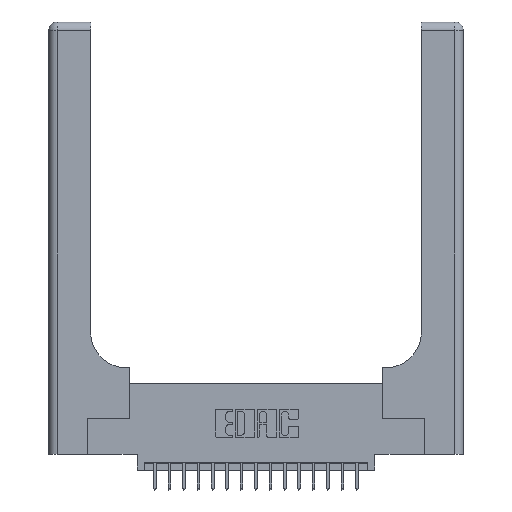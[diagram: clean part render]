
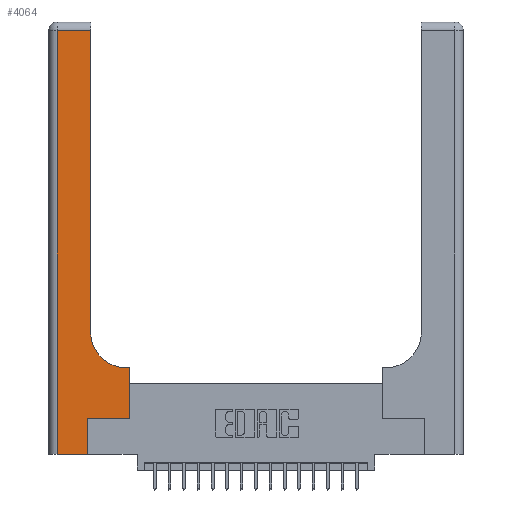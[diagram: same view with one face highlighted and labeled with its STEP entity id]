
A CAD part, top view. The second image highlights one B-rep face of the part: STEP entity #4064.
In plain terms, the highlighted planar face has unit normal (0, 0, 1).
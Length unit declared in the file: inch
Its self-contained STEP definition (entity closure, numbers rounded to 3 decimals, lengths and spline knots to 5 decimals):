
#77 = DIRECTION ( 'NONE',  ( -1., 0., 0. ) ) ;
#83 = VERTEX_POINT ( 'NONE', #14371 ) ;
#908 = LINE ( 'NONE', #13831, #20661 ) ;
#941 = VERTEX_POINT ( 'NONE', #7114 ) ;
#1025 = DIRECTION ( 'NONE',  ( 1., 0., 0. ) ) ;
#1724 = VECTOR ( 'NONE', #4347, 39.37008 ) ;
#1729 = ORIENTED_EDGE ( 'NONE', *, *, #18147, .T. ) ;
#2887 = VERTEX_POINT ( 'NONE', #5457 ) ;
#3178 = CIRCLE ( 'NONE', #10839, 0.25 ) ;
#3492 = CARTESIAN_POINT ( 'NONE',  ( 0.06, 0., 0.37 ) ) ;
#3884 = EDGE_CURVE ( 'NONE', #2887, #7071, #908, .T. ) ;
#3934 = DIRECTION ( 'NONE',  ( -1., 0., 0. ) ) ;
#4064 = ADVANCED_FACE ( 'NONE', ( #6858 ), #6968, .F. ) ;
#4347 = DIRECTION ( 'NONE',  ( 0., -1., 0. ) ) ;
#4430 = LINE ( 'NONE', #17370, #19109 ) ;
#4970 = DIRECTION ( 'NONE',  ( 1., 0., 0. ) ) ;
#5030 = CARTESIAN_POINT ( 'NONE',  ( 0.269, 0., 0.37 ) ) ;
#5044 = VECTOR ( 'NONE', #7420, 39.37008 ) ;
#5072 = CARTESIAN_POINT ( 'NONE',  ( 0.5585, 0.25, 0.37 ) ) ;
#5457 = CARTESIAN_POINT ( 'NONE',  ( 0.2915, 0.85, 0.37 ) ) ;
#5660 = EDGE_CURVE ( 'NONE', #83, #2887, #3178, .T. ) ;
#6353 = DIRECTION ( 'NONE',  ( 1., 0., 0. ) ) ;
#6858 = FACE_OUTER_BOUND ( 'NONE', #18296, .T. ) ;
#6968 = PLANE ( 'NONE',  #12203 ) ;
#7071 = VERTEX_POINT ( 'NONE', #13636 ) ;
#7099 = CARTESIAN_POINT ( 'NONE',  ( 0.5585, 0.6, 0.37 ) ) ;
#7114 = CARTESIAN_POINT ( 'NONE',  ( 0.269, 0., 0.37 ) ) ;
#7201 = CARTESIAN_POINT ( 'NONE',  ( 0.269, 0.25, 0.37 ) ) ;
#7228 = CARTESIAN_POINT ( 'NONE',  ( 0.5585, 0.25, 0.37 ) ) ;
#7420 = DIRECTION ( 'NONE',  ( 0., 1., 0. ) ) ;
#7601 = VECTOR ( 'NONE', #4970, 39.37008 ) ;
#8092 = CARTESIAN_POINT ( 'NONE',  ( 0.269, 0.25, 0.37 ) ) ;
#8152 = VECTOR ( 'NONE', #6353, 39.37008 ) ;
#8417 = ORIENTED_EDGE ( 'NONE', *, *, #9094, .T. ) ;
#9094 = EDGE_CURVE ( 'NONE', #11889, #12499, #9979, .T. ) ;
#9818 = DIRECTION ( 'NONE',  ( 0., 1., 0. ) ) ;
#9979 = LINE ( 'NONE', #8092, #7601 ) ;
#10362 = LINE ( 'NONE', #7228, #5044 ) ;
#10834 = CARTESIAN_POINT ( 'NONE',  ( 0.06, 2.94, 0.37 ) ) ;
#10839 = AXIS2_PLACEMENT_3D ( 'NONE', #18792, #12254, #1025 ) ;
#10935 = EDGE_CURVE ( 'NONE', #941, #11889, #13431, .T. ) ;
#11307 = ORIENTED_EDGE ( 'NONE', *, *, #3884, .T. ) ;
#11318 = VECTOR ( 'NONE', #9818, 39.37008 ) ;
#11889 = VERTEX_POINT ( 'NONE', #7201 ) ;
#11998 = ORIENTED_EDGE ( 'NONE', *, *, #13806, .T. ) ;
#12048 = ORIENTED_EDGE ( 'NONE', *, *, #18334, .T. ) ;
#12203 = AXIS2_PLACEMENT_3D ( 'NONE', #16662, #19724, #3934 ) ;
#12254 = DIRECTION ( 'NONE',  ( 0., 0., -1. ) ) ;
#12499 = VERTEX_POINT ( 'NONE', #5072 ) ;
#12564 = EDGE_CURVE ( 'NONE', #12499, #13043, #10362, .T. ) ;
#13043 = VERTEX_POINT ( 'NONE', #7099 ) ;
#13101 = CARTESIAN_POINT ( 'NONE',  ( 0., 2.94, 0.37 ) ) ;
#13136 = EDGE_CURVE ( 'NONE', #16213, #941, #18883, .T. ) ;
#13431 = LINE ( 'NONE', #5030, #11318 ) ;
#13636 = CARTESIAN_POINT ( 'NONE',  ( 0.2915, 2.94, 0.37 ) ) ;
#13804 = LINE ( 'NONE', #18660, #1724 ) ;
#13806 = EDGE_CURVE ( 'NONE', #13043, #83, #4430, .T. ) ;
#13831 = CARTESIAN_POINT ( 'NONE',  ( 0.2915, 3., 0.37 ) ) ;
#14371 = CARTESIAN_POINT ( 'NONE',  ( 0.5415, 0.6, 0.37 ) ) ;
#14786 = LINE ( 'NONE', #13101, #18176 ) ;
#15641 = ORIENTED_EDGE ( 'NONE', *, *, #12564, .T. ) ;
#15835 = ORIENTED_EDGE ( 'NONE', *, *, #10935, .T. ) ;
#16213 = VERTEX_POINT ( 'NONE', #3492 ) ;
#16662 = CARTESIAN_POINT ( 'NONE',  ( 0., 3., 0.37 ) ) ;
#17059 = DIRECTION ( 'NONE',  ( -1., 0., 0. ) ) ;
#17370 = CARTESIAN_POINT ( 'NONE',  ( 0.2915, 0.6, 0.37 ) ) ;
#17420 = CARTESIAN_POINT ( 'NONE',  ( 0., 0., 0.37 ) ) ;
#18147 = EDGE_CURVE ( 'NONE', #7071, #19428, #14786, .T. ) ;
#18176 = VECTOR ( 'NONE', #77, 39.37008 ) ;
#18296 = EDGE_LOOP ( 'NONE', ( #11307, #1729, #12048, #19522, #15835, #8417, #15641, #11998, #20678 ) ) ;
#18334 = EDGE_CURVE ( 'NONE', #19428, #16213, #13804, .T. ) ;
#18660 = CARTESIAN_POINT ( 'NONE',  ( 0.06, 3., 0.37 ) ) ;
#18792 = CARTESIAN_POINT ( 'NONE',  ( 0.5415, 0.85, 0.37 ) ) ;
#18883 = LINE ( 'NONE', #17420, #8152 ) ;
#19109 = VECTOR ( 'NONE', #17059, 39.37008 ) ;
#19428 = VERTEX_POINT ( 'NONE', #10834 ) ;
#19522 = ORIENTED_EDGE ( 'NONE', *, *, #13136, .T. ) ;
#19724 = DIRECTION ( 'NONE',  ( 0., 0., -1. ) ) ;
#20581 = DIRECTION ( 'NONE',  ( 0., 1., 0. ) ) ;
#20661 = VECTOR ( 'NONE', #20581, 39.37008 ) ;
#20678 = ORIENTED_EDGE ( 'NONE', *, *, #5660, .T. ) ;
